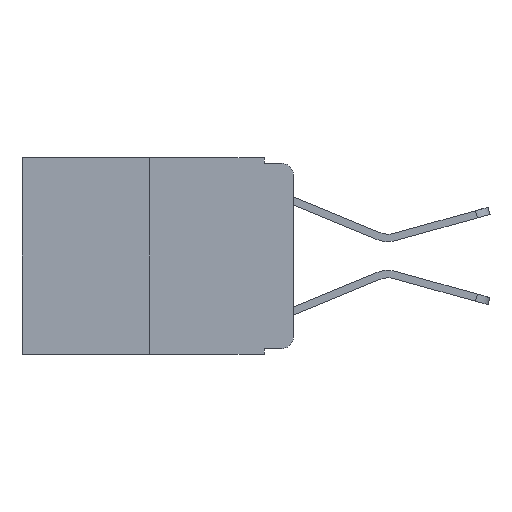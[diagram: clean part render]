
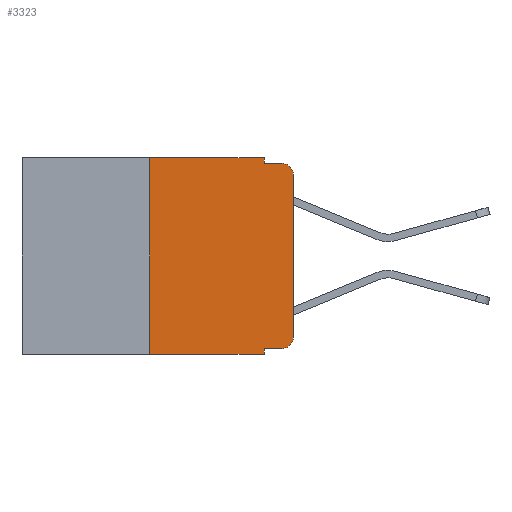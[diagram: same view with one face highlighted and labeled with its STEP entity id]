
A CAD part, left-side view. The second image highlights one B-rep face of the part: STEP entity #3323.
In plain terms, the highlighted planar face has unit normal (-1, 0, 0).
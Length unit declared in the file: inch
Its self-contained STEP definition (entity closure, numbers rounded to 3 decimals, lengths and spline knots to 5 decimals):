
#226 = EDGE_CURVE ( 'NONE', #9497, #1337, #10737, .T. ) ;
#611 = CARTESIAN_POINT ( 'NONE',  ( 0., 0.051, -0.333 ) ) ;
#704 = DIRECTION ( 'NONE',  ( 0., 0., -1. ) ) ;
#710 = EDGE_CURVE ( 'NONE', #7767, #3522, #10966, .T. ) ;
#760 = VERTEX_POINT ( 'NONE', #6341 ) ;
#823 = PLANE ( 'NONE',  #2205 ) ;
#1108 = VERTEX_POINT ( 'NONE', #4256 ) ;
#1337 = VERTEX_POINT ( 'NONE', #6982 ) ;
#1497 = VECTOR ( 'NONE', #7875, 39.37008 ) ;
#1719 = ORIENTED_EDGE ( 'NONE', *, *, #10803, .T. ) ;
#1772 = CARTESIAN_POINT ( 'NONE',  ( 0., 0.473, 0. ) ) ;
#1775 = LINE ( 'NONE', #3331, #10207 ) ;
#1909 = DIRECTION ( 'NONE',  ( 0., -1., 0. ) ) ;
#1915 = VERTEX_POINT ( 'NONE', #10478 ) ;
#1940 = DIRECTION ( 'NONE',  ( -1., 0., 0. ) ) ;
#1949 = EDGE_CURVE ( 'NONE', #760, #3522, #6841, .T. ) ;
#2076 = VECTOR ( 'NONE', #1909, 39.37008 ) ;
#2082 = EDGE_CURVE ( 'NONE', #1915, #5163, #3208, .T. ) ;
#2115 = EDGE_LOOP ( 'NONE', ( #6504, #1719, #9296, #10379, #9095, #10282, #9908, #10745, #2552, #4725 ) ) ;
#2205 = AXIS2_PLACEMENT_3D ( 'NONE', #9470, #4343, #8876 ) ;
#2552 = ORIENTED_EDGE ( 'NONE', *, *, #8382, .T. ) ;
#3003 = EDGE_CURVE ( 'NONE', #4806, #9497, #8625, .T. ) ;
#3008 = CARTESIAN_POINT ( 'NONE',  ( 0., 0.25, 0. ) ) ;
#3208 = CIRCLE ( 'NONE', #7897, 0.02 ) ;
#3323 = ADVANCED_FACE ( 'NONE', ( #5211 ), #823, .F. ) ;
#3331 = CARTESIAN_POINT ( 'NONE',  ( 0., 0.051, -0.01 ) ) ;
#3391 = EDGE_CURVE ( 'NONE', #5163, #1108, #10668, .T. ) ;
#3432 = DIRECTION ( 'NONE',  ( 0., 0., -1. ) ) ;
#3522 = VERTEX_POINT ( 'NONE', #7014 ) ;
#3590 = CARTESIAN_POINT ( 'NONE',  ( 0., 0.25, 0. ) ) ;
#3601 = VERTEX_POINT ( 'NONE', #10990 ) ;
#3671 = CARTESIAN_POINT ( 'NONE',  ( 0., 0., -0.313 ) ) ;
#4170 = VECTOR ( 'NONE', #704, 39.37008 ) ;
#4176 = DIRECTION ( 'NONE',  ( 0., -1., 0. ) ) ;
#4218 = CIRCLE ( 'NONE', #4876, 0.02 ) ;
#4256 = CARTESIAN_POINT ( 'NONE',  ( 0., 0., -0.03 ) ) ;
#4343 = DIRECTION ( 'NONE',  ( 1., 0., 0. ) ) ;
#4725 = ORIENTED_EDGE ( 'NONE', *, *, #2082, .T. ) ;
#4806 = VERTEX_POINT ( 'NONE', #3008 ) ;
#4876 = AXIS2_PLACEMENT_3D ( 'NONE', #7129, #1940, #7979 ) ;
#5163 = VERTEX_POINT ( 'NONE', #3671 ) ;
#5211 = FACE_OUTER_BOUND ( 'NONE', #2115, .T. ) ;
#5990 = CARTESIAN_POINT ( 'NONE',  ( 0., 0.051, 0. ) ) ;
#6176 = CARTESIAN_POINT ( 'NONE',  ( 0., 0.051, -0.333 ) ) ;
#6244 = DIRECTION ( 'NONE',  ( 0., -1., 0. ) ) ;
#6284 = LINE ( 'NONE', #611, #10314 ) ;
#6341 = CARTESIAN_POINT ( 'NONE',  ( 0., 0.25, -0.343 ) ) ;
#6504 = ORIENTED_EDGE ( 'NONE', *, *, #3391, .T. ) ;
#6841 = LINE ( 'NONE', #10226, #10828 ) ;
#6982 = CARTESIAN_POINT ( 'NONE',  ( 0., 0.051, -0.01 ) ) ;
#7014 = CARTESIAN_POINT ( 'NONE',  ( 0., 0.051, -0.343 ) ) ;
#7129 = CARTESIAN_POINT ( 'NONE',  ( 0., 0.02, -0.03 ) ) ;
#7551 = DIRECTION ( 'NONE',  ( 0., 0., -1. ) ) ;
#7767 = VERTEX_POINT ( 'NONE', #6176 ) ;
#7795 = EDGE_CURVE ( 'NONE', #760, #4806, #8375, .T. ) ;
#7875 = DIRECTION ( 'NONE',  ( 0., 0., 1. ) ) ;
#7897 = AXIS2_PLACEMENT_3D ( 'NONE', #10763, #10754, #7551 ) ;
#7979 = DIRECTION ( 'NONE',  ( 0., 0., -1. ) ) ;
#8208 = EDGE_CURVE ( 'NONE', #1337, #3601, #1775, .T. ) ;
#8375 = LINE ( 'NONE', #3590, #1497 ) ;
#8382 = EDGE_CURVE ( 'NONE', #7767, #1915, #6284, .T. ) ;
#8617 = VECTOR ( 'NONE', #9506, 39.37008 ) ;
#8625 = LINE ( 'NONE', #1772, #2076 ) ;
#8876 = DIRECTION ( 'NONE',  ( 0., 0., -1. ) ) ;
#8911 = VECTOR ( 'NONE', #3432, 39.37008 ) ;
#9095 = ORIENTED_EDGE ( 'NONE', *, *, #3003, .F. ) ;
#9279 = CARTESIAN_POINT ( 'NONE',  ( 0., 0.051, 0. ) ) ;
#9296 = ORIENTED_EDGE ( 'NONE', *, *, #8208, .F. ) ;
#9470 = CARTESIAN_POINT ( 'NONE',  ( 0., 0.473, 0. ) ) ;
#9497 = VERTEX_POINT ( 'NONE', #9279 ) ;
#9506 = DIRECTION ( 'NONE',  ( 0., 0., 1. ) ) ;
#9908 = ORIENTED_EDGE ( 'NONE', *, *, #1949, .T. ) ;
#10207 = VECTOR ( 'NONE', #4176, 39.37008 ) ;
#10226 = CARTESIAN_POINT ( 'NONE',  ( 0., 0.473, -0.343 ) ) ;
#10282 = ORIENTED_EDGE ( 'NONE', *, *, #7795, .F. ) ;
#10314 = VECTOR ( 'NONE', #10747, 39.37008 ) ;
#10379 = ORIENTED_EDGE ( 'NONE', *, *, #226, .F. ) ;
#10478 = CARTESIAN_POINT ( 'NONE',  ( 0., 0.02, -0.333 ) ) ;
#10486 = CARTESIAN_POINT ( 'NONE',  ( 0., 0.051, 0. ) ) ;
#10668 = LINE ( 'NONE', #10928, #8617 ) ;
#10737 = LINE ( 'NONE', #10486, #4170 ) ;
#10745 = ORIENTED_EDGE ( 'NONE', *, *, #710, .F. ) ;
#10747 = DIRECTION ( 'NONE',  ( 0., -1., 0. ) ) ;
#10754 = DIRECTION ( 'NONE',  ( -1., 0., 0. ) ) ;
#10763 = CARTESIAN_POINT ( 'NONE',  ( 0., 0.02, -0.313 ) ) ;
#10803 = EDGE_CURVE ( 'NONE', #1108, #3601, #4218, .T. ) ;
#10828 = VECTOR ( 'NONE', #6244, 39.37008 ) ;
#10928 = CARTESIAN_POINT ( 'NONE',  ( 0., 0., 0. ) ) ;
#10966 = LINE ( 'NONE', #5990, #8911 ) ;
#10990 = CARTESIAN_POINT ( 'NONE',  ( 0., 0.02, -0.01 ) ) ;
